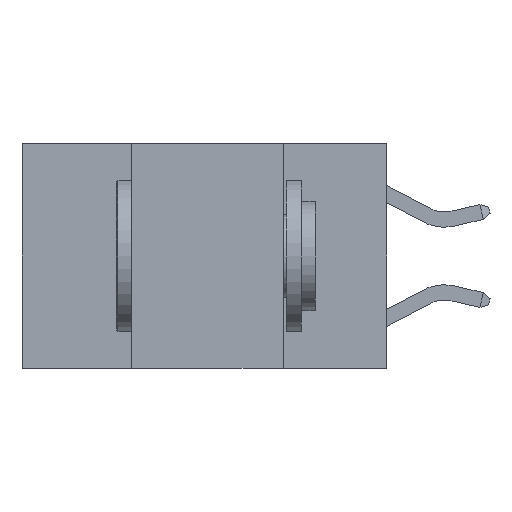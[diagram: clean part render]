
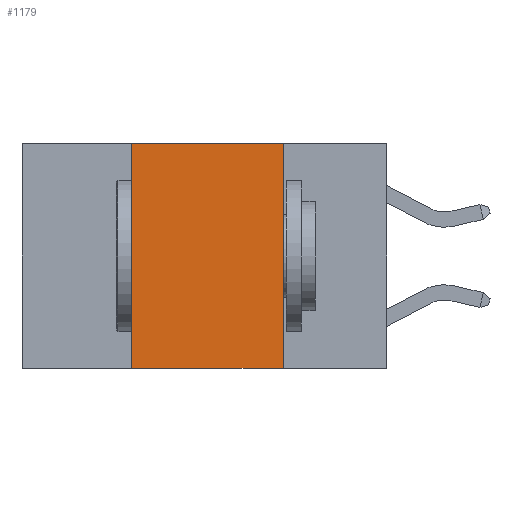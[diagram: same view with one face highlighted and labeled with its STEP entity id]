
A CAD part, left-side view. The second image highlights one B-rep face of the part: STEP entity #1179.
In plain terms, the highlighted planar face has unit normal (-1, 0, 0).
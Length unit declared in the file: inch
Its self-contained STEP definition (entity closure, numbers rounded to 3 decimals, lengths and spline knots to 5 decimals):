
#506 = CARTESIAN_POINT ( 'NONE',  ( 0., 0.17, 0. ) ) ;
#533 = DIRECTION ( 'NONE',  ( 0., 0., 1. ) ) ;
#845 = ORIENTED_EDGE ( 'NONE', *, *, #13144, .F. ) ;
#1179 = ADVANCED_FACE ( 'NONE', ( #10769 ), #3826, .F. ) ;
#1219 = ORIENTED_EDGE ( 'NONE', *, *, #12011, .F. ) ;
#2552 = LINE ( 'NONE', #506, #10085 ) ;
#2759 = ORIENTED_EDGE ( 'NONE', *, *, #4912, .T. ) ;
#3189 = VERTEX_POINT ( 'NONE', #3399 ) ;
#3305 = ORIENTED_EDGE ( 'NONE', *, *, #6520, .F. ) ;
#3399 = CARTESIAN_POINT ( 'NONE',  ( 0., 0.42, 0. ) ) ;
#3826 = PLANE ( 'NONE',  #7213 ) ;
#4231 = CARTESIAN_POINT ( 'NONE',  ( 0., 0.17, 0. ) ) ;
#4428 = CARTESIAN_POINT ( 'NONE',  ( 0., 0.42, -0.37 ) ) ;
#4676 = VECTOR ( 'NONE', #11144, 39.37008 ) ;
#4768 = VECTOR ( 'NONE', #7938, 39.37008 ) ;
#4912 = EDGE_CURVE ( 'NONE', #11288, #8157, #9007, .T. ) ;
#5160 = CARTESIAN_POINT ( 'NONE',  ( 0., 0.6, 0. ) ) ;
#5592 = LINE ( 'NONE', #6671, #7116 ) ;
#6242 = VERTEX_POINT ( 'NONE', #4231 ) ;
#6520 = EDGE_CURVE ( 'NONE', #11288, #3189, #5592, .T. ) ;
#6671 = CARTESIAN_POINT ( 'NONE',  ( 0., 0.42, 0. ) ) ;
#6914 = DIRECTION ( 'NONE',  ( 1., 0., 0. ) ) ;
#7116 = VECTOR ( 'NONE', #533, 39.37008 ) ;
#7213 = AXIS2_PLACEMENT_3D ( 'NONE', #10831, #6914, #11836 ) ;
#7218 = CARTESIAN_POINT ( 'NONE',  ( 0., 0.17, -0.37 ) ) ;
#7938 = DIRECTION ( 'NONE',  ( 0., -1., 0. ) ) ;
#8157 = VERTEX_POINT ( 'NONE', #7218 ) ;
#9007 = LINE ( 'NONE', #13275, #4676 ) ;
#9705 = EDGE_LOOP ( 'NONE', ( #845, #1219, #3305, #2759 ) ) ;
#10085 = VECTOR ( 'NONE', #13035, 39.37008 ) ;
#10250 = LINE ( 'NONE', #5160, #4768 ) ;
#10769 = FACE_OUTER_BOUND ( 'NONE', #9705, .T. ) ;
#10831 = CARTESIAN_POINT ( 'NONE',  ( 0., 0.6, 0. ) ) ;
#11144 = DIRECTION ( 'NONE',  ( 0., -1., 0. ) ) ;
#11288 = VERTEX_POINT ( 'NONE', #4428 ) ;
#11836 = DIRECTION ( 'NONE',  ( 0., 0., -1. ) ) ;
#12011 = EDGE_CURVE ( 'NONE', #3189, #6242, #10250, .T. ) ;
#13035 = DIRECTION ( 'NONE',  ( 0., 0., -1. ) ) ;
#13144 = EDGE_CURVE ( 'NONE', #6242, #8157, #2552, .T. ) ;
#13275 = CARTESIAN_POINT ( 'NONE',  ( 0., 0.6, -0.37 ) ) ;
